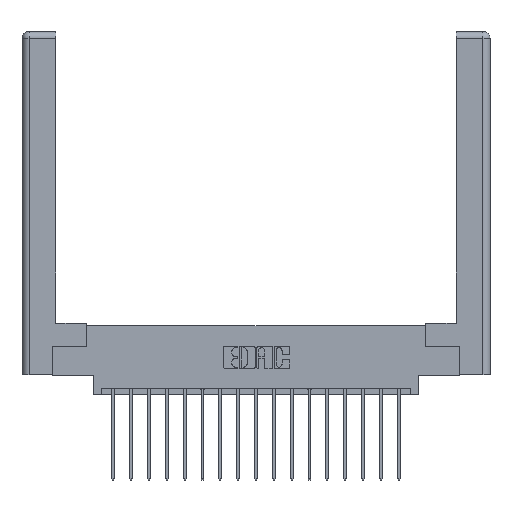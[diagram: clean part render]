
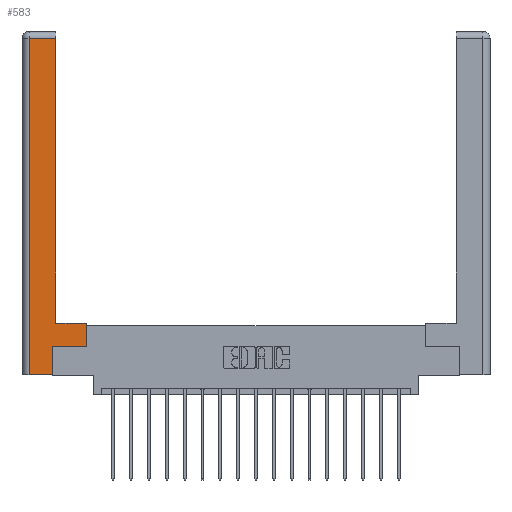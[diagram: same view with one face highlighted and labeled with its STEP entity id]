
A CAD part, top view. The second image highlights one B-rep face of the part: STEP entity #583.
In plain terms, the highlighted planar face has unit normal (0, 0, 1).
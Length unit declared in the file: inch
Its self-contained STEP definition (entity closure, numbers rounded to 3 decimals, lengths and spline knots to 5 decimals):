
#168 = ORIENTED_EDGE ( 'NONE', *, *, #7989, .T. ) ;
#583 = ADVANCED_FACE ( 'NONE', ( #14657 ), #15755, .F. ) ;
#688 = LINE ( 'NONE', #13799, #18829 ) ;
#740 = CARTESIAN_POINT ( 'NONE',  ( 0., 0., 0. ) ) ;
#866 = DIRECTION ( 'NONE',  ( 0., 0., -1. ) ) ;
#987 = VERTEX_POINT ( 'NONE', #17134 ) ;
#1120 = DIRECTION ( 'NONE',  ( 0., 1., 0. ) ) ;
#1380 = AXIS2_PLACEMENT_3D ( 'NONE', #740, #866, #11152 ) ;
#2085 = VERTEX_POINT ( 'NONE', #5656 ) ;
#2148 = CARTESIAN_POINT ( 'NONE',  ( 0.265, 0.245, 0. ) ) ;
#2187 = LINE ( 'NONE', #12081, #6648 ) ;
#3385 = ORIENTED_EDGE ( 'NONE', *, *, #16883, .T. ) ;
#4214 = LINE ( 'NONE', #2148, #12353 ) ;
#4342 = CARTESIAN_POINT ( 'NONE',  ( 0.565, 0.245, 0. ) ) ;
#4584 = ORIENTED_EDGE ( 'NONE', *, *, #11523, .T. ) ;
#4660 = LINE ( 'NONE', #17806, #11881 ) ;
#4752 = DIRECTION ( 'NONE',  ( 0., -1., 0. ) ) ;
#4945 = CARTESIAN_POINT ( 'NONE',  ( 0.295, 3., 0. ) ) ;
#5372 = EDGE_CURVE ( 'NONE', #10426, #8530, #2187, .T. ) ;
#5656 = CARTESIAN_POINT ( 'NONE',  ( 0.295, 2.94, 0. ) ) ;
#6489 = CARTESIAN_POINT ( 'NONE',  ( 0.265, 0., 0. ) ) ;
#6648 = VECTOR ( 'NONE', #13692, 39.37008 ) ;
#6763 = CARTESIAN_POINT ( 'NONE',  ( 0.0615, 0., 0. ) ) ;
#6964 = EDGE_CURVE ( 'NONE', #14266, #987, #13759, .T. ) ;
#7199 = DIRECTION ( 'NONE',  ( 1., 0., 0. ) ) ;
#7380 = VERTEX_POINT ( 'NONE', #15972 ) ;
#7465 = EDGE_CURVE ( 'NONE', #8530, #17052, #4660, .T. ) ;
#7524 = LINE ( 'NONE', #17534, #18868 ) ;
#7763 = ORIENTED_EDGE ( 'NONE', *, *, #6964, .T. ) ;
#7989 = EDGE_CURVE ( 'NONE', #15506, #14266, #688, .T. ) ;
#8530 = VERTEX_POINT ( 'NONE', #16243 ) ;
#8537 = VECTOR ( 'NONE', #12607, 39.37008 ) ;
#8749 = LINE ( 'NONE', #16777, #8537 ) ;
#9686 = ORIENTED_EDGE ( 'NONE', *, *, #19003, .T. ) ;
#10112 = ORIENTED_EDGE ( 'NONE', *, *, #5372, .T. ) ;
#10426 = VERTEX_POINT ( 'NONE', #4342 ) ;
#11152 = DIRECTION ( 'NONE',  ( -1., 0., 0. ) ) ;
#11523 = EDGE_CURVE ( 'NONE', #7380, #10426, #7524, .T. ) ;
#11881 = VECTOR ( 'NONE', #16384, 39.37008 ) ;
#12081 = CARTESIAN_POINT ( 'NONE',  ( 0.565, 0.45, 0. ) ) ;
#12353 = VECTOR ( 'NONE', #1120, 39.37008 ) ;
#12607 = DIRECTION ( 'NONE',  ( -1., 0., 0. ) ) ;
#13099 = EDGE_LOOP ( 'NONE', ( #3385, #9686, #168, #7763, #16043, #4584, #10112, #14216 ) ) ;
#13692 = DIRECTION ( 'NONE',  ( 0., 1., 0. ) ) ;
#13759 = LINE ( 'NONE', #6489, #14227 ) ;
#13799 = CARTESIAN_POINT ( 'NONE',  ( 0.0615, 0., 0. ) ) ;
#14216 = ORIENTED_EDGE ( 'NONE', *, *, #7465, .T. ) ;
#14227 = VECTOR ( 'NONE', #16973, 39.37008 ) ;
#14266 = VERTEX_POINT ( 'NONE', #6763 ) ;
#14657 = FACE_OUTER_BOUND ( 'NONE', #13099, .T. ) ;
#15506 = VERTEX_POINT ( 'NONE', #18306 ) ;
#15755 = PLANE ( 'NONE',  #1380 ) ;
#15887 = LINE ( 'NONE', #4945, #17279 ) ;
#15972 = CARTESIAN_POINT ( 'NONE',  ( 0.265, 0.245, 0. ) ) ;
#16043 = ORIENTED_EDGE ( 'NONE', *, *, #19125, .T. ) ;
#16243 = CARTESIAN_POINT ( 'NONE',  ( 0.565, 0.45, 0. ) ) ;
#16384 = DIRECTION ( 'NONE',  ( -1., 0., 0. ) ) ;
#16777 = CARTESIAN_POINT ( 'NONE',  ( 0.0615, 2.94, 0. ) ) ;
#16883 = EDGE_CURVE ( 'NONE', #17052, #2085, #15887, .T. ) ;
#16973 = DIRECTION ( 'NONE',  ( 1., 0., 0. ) ) ;
#17052 = VERTEX_POINT ( 'NONE', #18381 ) ;
#17134 = CARTESIAN_POINT ( 'NONE',  ( 0.265, 0., 0. ) ) ;
#17279 = VECTOR ( 'NONE', #18393, 39.37008 ) ;
#17534 = CARTESIAN_POINT ( 'NONE',  ( 0.565, 0.245, 0. ) ) ;
#17806 = CARTESIAN_POINT ( 'NONE',  ( 0.295, 0.45, 0. ) ) ;
#18306 = CARTESIAN_POINT ( 'NONE',  ( 0.0615, 2.94, 0. ) ) ;
#18381 = CARTESIAN_POINT ( 'NONE',  ( 0.295, 0.45, 0. ) ) ;
#18393 = DIRECTION ( 'NONE',  ( 0., 1., 0. ) ) ;
#18829 = VECTOR ( 'NONE', #4752, 39.37008 ) ;
#18868 = VECTOR ( 'NONE', #7199, 39.37008 ) ;
#19003 = EDGE_CURVE ( 'NONE', #2085, #15506, #8749, .T. ) ;
#19125 = EDGE_CURVE ( 'NONE', #987, #7380, #4214, .T. ) ;
